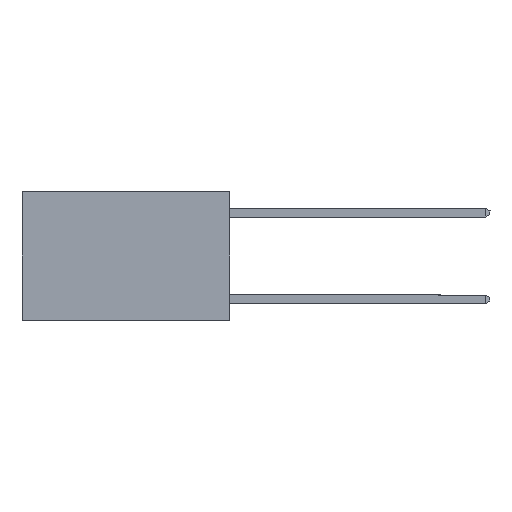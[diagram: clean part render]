
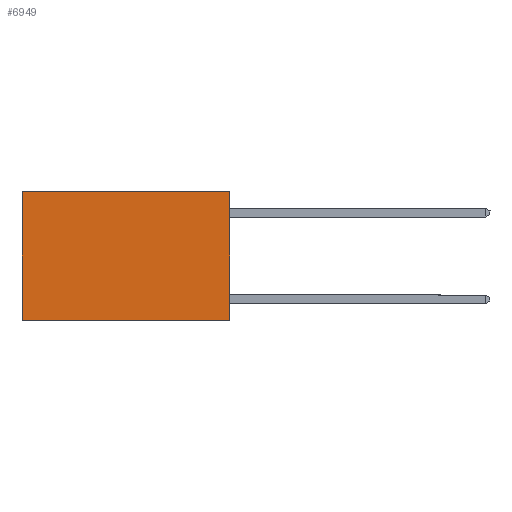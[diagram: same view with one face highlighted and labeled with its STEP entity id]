
A CAD part, left-side view. The second image highlights one B-rep face of the part: STEP entity #6949.
In plain terms, the highlighted planar face has unit normal (-1, 0, 0).
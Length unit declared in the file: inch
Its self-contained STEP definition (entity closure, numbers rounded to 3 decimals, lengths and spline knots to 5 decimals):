
#89 = ORIENTED_EDGE ( 'NONE', *, *, #16176, .F. ) ;
#144 = CARTESIAN_POINT ( 'NONE',  ( 0.2625, 0., -0.37 ) ) ;
#567 = VERTEX_POINT ( 'NONE', #4297 ) ;
#660 = CARTESIAN_POINT ( 'NONE',  ( 0.2625, 0., 0. ) ) ;
#897 = CARTESIAN_POINT ( 'NONE',  ( 0.2625, 0., 0. ) ) ;
#2045 = ORIENTED_EDGE ( 'NONE', *, *, #13894, .T. ) ;
#2786 = AXIS2_PLACEMENT_3D ( 'NONE', #660, #15911, #7625 ) ;
#3371 = ORIENTED_EDGE ( 'NONE', *, *, #10972, .F. ) ;
#3608 = LINE ( 'NONE', #13537, #14622 ) ;
#4297 = CARTESIAN_POINT ( 'NONE',  ( 0.2625, 0., 0. ) ) ;
#5417 = EDGE_CURVE ( 'NONE', #567, #15219, #16682, .T. ) ;
#5567 = EDGE_LOOP ( 'NONE', ( #2045, #3371, #89, #17747 ) ) ;
#6243 = PLANE ( 'NONE',  #2786 ) ;
#6629 = LINE ( 'NONE', #7083, #17589 ) ;
#6949 = ADVANCED_FACE ( 'NONE', ( #17252 ), #6243, .F. ) ;
#7083 = CARTESIAN_POINT ( 'NONE',  ( 0.2625, 0., 0. ) ) ;
#7625 = DIRECTION ( 'NONE',  ( 0., 0., -1. ) ) ;
#8423 = CARTESIAN_POINT ( 'NONE',  ( 0.2625, 0.6, 0. ) ) ;
#9186 = DIRECTION ( 'NONE',  ( 0., 1., 0. ) ) ;
#9352 = VECTOR ( 'NONE', #9186, 39.37008 ) ;
#9954 = CARTESIAN_POINT ( 'NONE',  ( 0.2625, 0.6, 0. ) ) ;
#10366 = LINE ( 'NONE', #9954, #17257 ) ;
#10972 = EDGE_CURVE ( 'NONE', #16827, #13295, #3608, .T. ) ;
#11370 = DIRECTION ( 'NONE',  ( 0., 0., -1. ) ) ;
#12220 = DIRECTION ( 'NONE',  ( 0., 1., 0. ) ) ;
#13295 = VERTEX_POINT ( 'NONE', #14288 ) ;
#13537 = CARTESIAN_POINT ( 'NONE',  ( 0.2625, 0., -0.37 ) ) ;
#13894 = EDGE_CURVE ( 'NONE', #15219, #13295, #10366, .T. ) ;
#14288 = CARTESIAN_POINT ( 'NONE',  ( 0.2625, 0.6, -0.37 ) ) ;
#14622 = VECTOR ( 'NONE', #12220, 39.37008 ) ;
#15219 = VERTEX_POINT ( 'NONE', #8423 ) ;
#15911 = DIRECTION ( 'NONE',  ( 1., 0., 0. ) ) ;
#16176 = EDGE_CURVE ( 'NONE', #567, #16827, #6629, .T. ) ;
#16682 = LINE ( 'NONE', #897, #9352 ) ;
#16711 = DIRECTION ( 'NONE',  ( 0., 0., -1. ) ) ;
#16827 = VERTEX_POINT ( 'NONE', #144 ) ;
#17252 = FACE_OUTER_BOUND ( 'NONE', #5567, .T. ) ;
#17257 = VECTOR ( 'NONE', #11370, 39.37008 ) ;
#17589 = VECTOR ( 'NONE', #16711, 39.37008 ) ;
#17747 = ORIENTED_EDGE ( 'NONE', *, *, #5417, .T. ) ;
